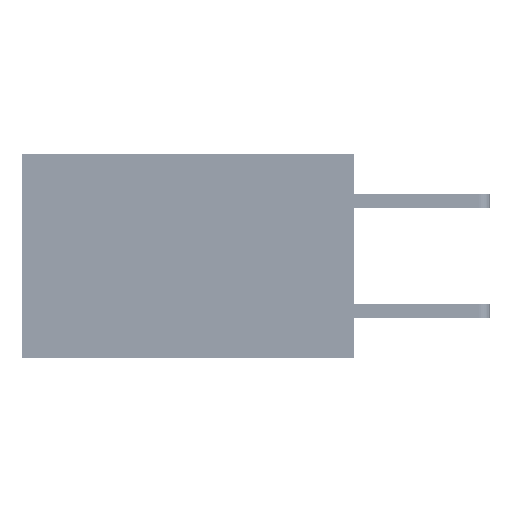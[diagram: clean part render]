
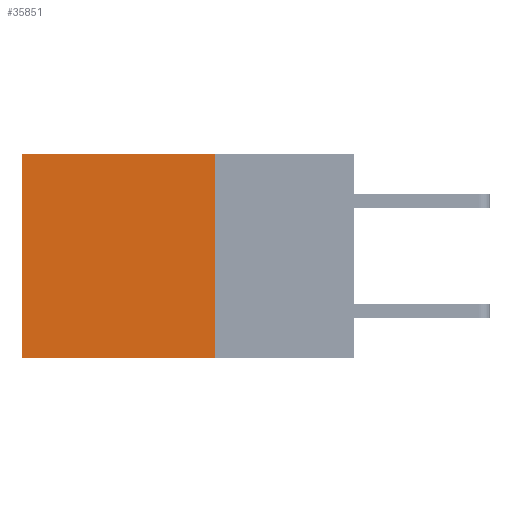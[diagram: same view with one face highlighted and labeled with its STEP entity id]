
A CAD part, left-side view. The second image highlights one B-rep face of the part: STEP entity #35851.
In plain terms, the highlighted planar face has unit normal (-1, 0, 0).
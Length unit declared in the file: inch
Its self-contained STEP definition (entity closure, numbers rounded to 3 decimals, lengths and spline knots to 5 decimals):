
#558 = FACE_OUTER_BOUND ( 'NONE', #3371, .T. ) ;
#989 = DIRECTION ( 'NONE',  ( 0., 1., 0. ) ) ;
#1039 = VERTEX_POINT ( 'NONE', #1909 ) ;
#1909 = CARTESIAN_POINT ( 'NONE',  ( 0.2875, 0.25, 0. ) ) ;
#2208 = PLANE ( 'NONE',  #33875 ) ;
#3371 = EDGE_LOOP ( 'NONE', ( #18870, #27958, #21296, #24797 ) ) ;
#3763 = VERTEX_POINT ( 'NONE', #35652 ) ;
#4132 = LINE ( 'NONE', #19407, #35633 ) ;
#5193 = LINE ( 'NONE', #35921, #22678 ) ;
#8569 = EDGE_CURVE ( 'NONE', #13415, #27000, #4132, .T. ) ;
#11984 = VECTOR ( 'NONE', #36839, 39.37008 ) ;
#12992 = VECTOR ( 'NONE', #33806, 39.37008 ) ;
#13415 = VERTEX_POINT ( 'NONE', #28473 ) ;
#14381 = DIRECTION ( 'NONE',  ( 0., 0., -1. ) ) ;
#14506 = CARTESIAN_POINT ( 'NONE',  ( 0.2875, 0.25, 0. ) ) ;
#17317 = DIRECTION ( 'NONE',  ( 0., 1., 0. ) ) ;
#18870 = ORIENTED_EDGE ( 'NONE', *, *, #32247, .T. ) ;
#19407 = CARTESIAN_POINT ( 'NONE',  ( 0.2875, 0.25, -0.37 ) ) ;
#19470 = LINE ( 'NONE', #27443, #11984 ) ;
#21296 = ORIENTED_EDGE ( 'NONE', *, *, #21366, .F. ) ;
#21366 = EDGE_CURVE ( 'NONE', #1039, #13415, #26502, .T. ) ;
#22678 = VECTOR ( 'NONE', #989, 39.37008 ) ;
#24797 = ORIENTED_EDGE ( 'NONE', *, *, #34323, .T. ) ;
#26502 = LINE ( 'NONE', #40069, #12992 ) ;
#27000 = VERTEX_POINT ( 'NONE', #35585 ) ;
#27443 = CARTESIAN_POINT ( 'NONE',  ( 0.2875, 0.6, 0. ) ) ;
#27958 = ORIENTED_EDGE ( 'NONE', *, *, #8569, .F. ) ;
#28473 = CARTESIAN_POINT ( 'NONE',  ( 0.2875, 0.25, -0.37 ) ) ;
#32247 = EDGE_CURVE ( 'NONE', #3763, #27000, #19470, .T. ) ;
#33806 = DIRECTION ( 'NONE',  ( 0., 0., -1. ) ) ;
#33875 = AXIS2_PLACEMENT_3D ( 'NONE', #14506, #40206, #14381 ) ;
#34323 = EDGE_CURVE ( 'NONE', #1039, #3763, #5193, .T. ) ;
#35585 = CARTESIAN_POINT ( 'NONE',  ( 0.2875, 0.6, -0.37 ) ) ;
#35633 = VECTOR ( 'NONE', #17317, 39.37008 ) ;
#35652 = CARTESIAN_POINT ( 'NONE',  ( 0.2875, 0.6, 0. ) ) ;
#35851 = ADVANCED_FACE ( 'NONE', ( #558 ), #2208, .F. ) ;
#35921 = CARTESIAN_POINT ( 'NONE',  ( 0.2875, 0.25, 0. ) ) ;
#36839 = DIRECTION ( 'NONE',  ( 0., 0., -1. ) ) ;
#40069 = CARTESIAN_POINT ( 'NONE',  ( 0.2875, 0.25, 0. ) ) ;
#40206 = DIRECTION ( 'NONE',  ( 1., 0., 0. ) ) ;
